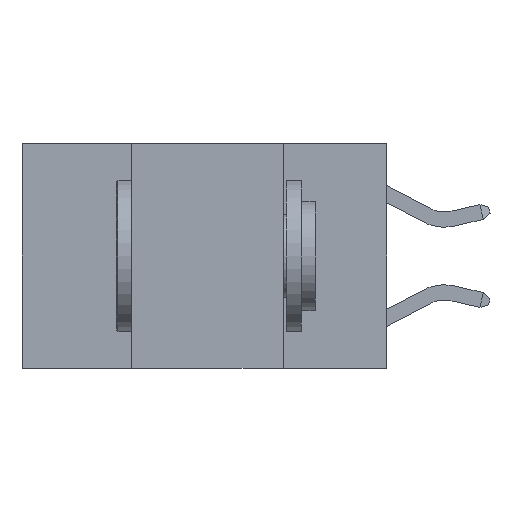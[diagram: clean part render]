
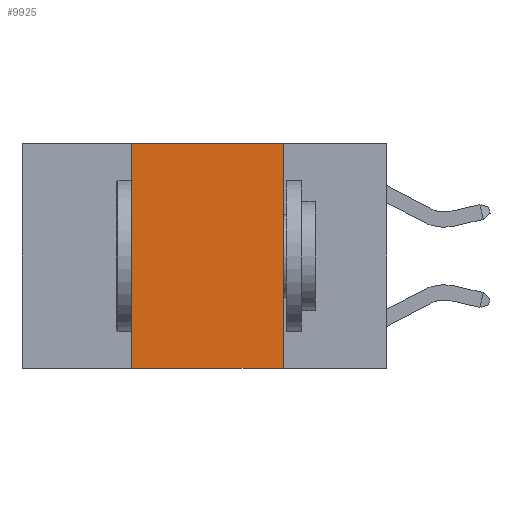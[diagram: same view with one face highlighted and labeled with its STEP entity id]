
A CAD part, left-side view. The second image highlights one B-rep face of the part: STEP entity #9925.
In plain terms, the highlighted planar face has unit normal (-1, 0, 0).
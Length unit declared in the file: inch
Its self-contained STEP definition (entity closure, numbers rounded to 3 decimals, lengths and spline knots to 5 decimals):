
#868 = EDGE_CURVE ( 'NONE', #13836, #3951, #8114, .T. ) ;
#1617 = VERTEX_POINT ( 'NONE', #9713 ) ;
#2067 = PLANE ( 'NONE',  #5472 ) ;
#2607 = VERTEX_POINT ( 'NONE', #14165 ) ;
#2811 = VECTOR ( 'NONE', #13022, 39.37008 ) ;
#3951 = VERTEX_POINT ( 'NONE', #16247 ) ;
#4229 = ORIENTED_EDGE ( 'NONE', *, *, #10699, .F. ) ;
#4817 = ORIENTED_EDGE ( 'NONE', *, *, #868, .F. ) ;
#5472 = AXIS2_PLACEMENT_3D ( 'NONE', #12312, #14826, #7322 ) ;
#5680 = ORIENTED_EDGE ( 'NONE', *, *, #8131, .F. ) ;
#5928 = ORIENTED_EDGE ( 'NONE', *, *, #8125, .T. ) ;
#6297 = LINE ( 'NONE', #8053, #2811 ) ;
#6758 = DIRECTION ( 'NONE',  ( 0., 0., 1. ) ) ;
#7322 = DIRECTION ( 'NONE',  ( 0., 0., -1. ) ) ;
#7688 = CARTESIAN_POINT ( 'NONE',  ( 0., 0.17, 0. ) ) ;
#8053 = CARTESIAN_POINT ( 'NONE',  ( 0., 0.6, -0.37 ) ) ;
#8114 = LINE ( 'NONE', #10344, #13979 ) ;
#8125 = EDGE_CURVE ( 'NONE', #1617, #2607, #6297, .T. ) ;
#8131 = EDGE_CURVE ( 'NONE', #1617, #13836, #12579, .T. ) ;
#8551 = EDGE_LOOP ( 'NONE', ( #4229, #4817, #5680, #5928 ) ) ;
#9319 = CARTESIAN_POINT ( 'NONE',  ( 0., 0.42, 0. ) ) ;
#9652 = CARTESIAN_POINT ( 'NONE',  ( 0., 0.42, 0. ) ) ;
#9713 = CARTESIAN_POINT ( 'NONE',  ( 0., 0.42, -0.37 ) ) ;
#9925 = ADVANCED_FACE ( 'NONE', ( #11363 ), #2067, .F. ) ;
#10344 = CARTESIAN_POINT ( 'NONE',  ( 0., 0.6, 0. ) ) ;
#10429 = DIRECTION ( 'NONE',  ( 0., -1., 0. ) ) ;
#10699 = EDGE_CURVE ( 'NONE', #3951, #2607, #12128, .T. ) ;
#11363 = FACE_OUTER_BOUND ( 'NONE', #8551, .T. ) ;
#12128 = LINE ( 'NONE', #7688, #15073 ) ;
#12312 = CARTESIAN_POINT ( 'NONE',  ( 0., 0.6, 0. ) ) ;
#12579 = LINE ( 'NONE', #9319, #15495 ) ;
#13022 = DIRECTION ( 'NONE',  ( 0., -1., 0. ) ) ;
#13836 = VERTEX_POINT ( 'NONE', #9652 ) ;
#13979 = VECTOR ( 'NONE', #10429, 39.37008 ) ;
#14165 = CARTESIAN_POINT ( 'NONE',  ( 0., 0.17, -0.37 ) ) ;
#14826 = DIRECTION ( 'NONE',  ( 1., 0., 0. ) ) ;
#15073 = VECTOR ( 'NONE', #16421, 39.37008 ) ;
#15495 = VECTOR ( 'NONE', #6758, 39.37008 ) ;
#16247 = CARTESIAN_POINT ( 'NONE',  ( 0., 0.17, 0. ) ) ;
#16421 = DIRECTION ( 'NONE',  ( 0., 0., -1. ) ) ;
